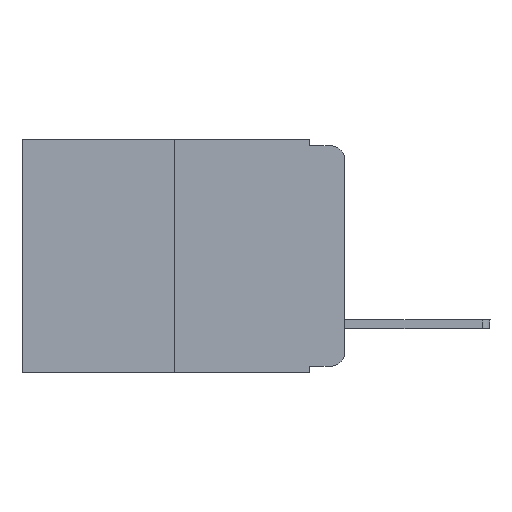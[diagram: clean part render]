
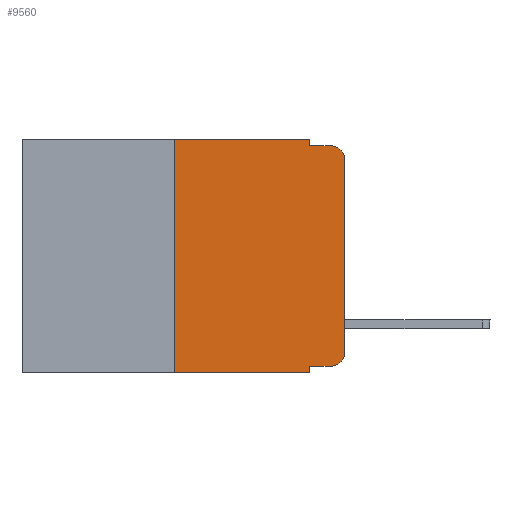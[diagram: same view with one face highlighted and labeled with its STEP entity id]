
A CAD part, left-side view. The second image highlights one B-rep face of the part: STEP entity #9560.
In plain terms, the highlighted planar face has unit normal (-1, 0, 0).
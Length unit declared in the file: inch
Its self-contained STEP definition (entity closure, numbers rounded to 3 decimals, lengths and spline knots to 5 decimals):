
#354 = LINE ( 'NONE', #13941, #14107 ) ;
#539 = CARTESIAN_POINT ( 'NONE',  ( 0., 0., -0.313 ) ) ;
#550 = ORIENTED_EDGE ( 'NONE', *, *, #10708, .F. ) ;
#658 = ORIENTED_EDGE ( 'NONE', *, *, #13967, .T. ) ;
#851 = VERTEX_POINT ( 'NONE', #7822 ) ;
#1199 = VECTOR ( 'NONE', #11061, 39.37008 ) ;
#1207 = CIRCLE ( 'NONE', #9537, 0.02 ) ;
#1257 = LINE ( 'NONE', #5520, #4127 ) ;
#1482 = LINE ( 'NONE', #12914, #13289 ) ;
#1785 = LINE ( 'NONE', #14321, #1199 ) ;
#2118 = DIRECTION ( 'NONE',  ( 0., -1., 0. ) ) ;
#2316 = DIRECTION ( 'NONE',  ( 0., 0., -1. ) ) ;
#2577 = DIRECTION ( 'NONE',  ( 0., -1., 0. ) ) ;
#2596 = DIRECTION ( 'NONE',  ( 0., 0., 1. ) ) ;
#2647 = EDGE_LOOP ( 'NONE', ( #3524, #3089, #8694, #12644, #550, #14440, #658, #9590, #8175, #4235 ) ) ;
#2706 = AXIS2_PLACEMENT_3D ( 'NONE', #4017, #4155, #7640 ) ;
#3079 = VERTEX_POINT ( 'NONE', #6579 ) ;
#3089 = ORIENTED_EDGE ( 'NONE', *, *, #12311, .T. ) ;
#3452 = DIRECTION ( 'NONE',  ( 0., 0., -1. ) ) ;
#3524 = ORIENTED_EDGE ( 'NONE', *, *, #10540, .T. ) ;
#3724 = LINE ( 'NONE', #10770, #3833 ) ;
#3833 = VECTOR ( 'NONE', #2596, 39.37008 ) ;
#4017 = CARTESIAN_POINT ( 'NONE',  ( 0., 0.02, -0.03 ) ) ;
#4127 = VECTOR ( 'NONE', #2316, 39.37008 ) ;
#4155 = DIRECTION ( 'NONE',  ( -1., 0., 0. ) ) ;
#4235 = ORIENTED_EDGE ( 'NONE', *, *, #9045, .T. ) ;
#4720 = FACE_OUTER_BOUND ( 'NONE', #2647, .T. ) ;
#4818 = LINE ( 'NONE', #13850, #9409 ) ;
#5110 = CARTESIAN_POINT ( 'NONE',  ( 0., 0.02, -0.01 ) ) ;
#5168 = VERTEX_POINT ( 'NONE', #10746 ) ;
#5216 = VERTEX_POINT ( 'NONE', #5110 ) ;
#5265 = CARTESIAN_POINT ( 'NONE',  ( 0., 0.051, -0.333 ) ) ;
#5301 = EDGE_CURVE ( 'NONE', #14570, #5216, #8800, .T. ) ;
#5520 = CARTESIAN_POINT ( 'NONE',  ( 0., 0.051, 0. ) ) ;
#6579 = CARTESIAN_POINT ( 'NONE',  ( 0., 0.051, -0.343 ) ) ;
#7280 = DIRECTION ( 'NONE',  ( 0., 0., 1. ) ) ;
#7375 = VECTOR ( 'NONE', #2118, 39.37008 ) ;
#7640 = DIRECTION ( 'NONE',  ( 0., 0., -1. ) ) ;
#7822 = CARTESIAN_POINT ( 'NONE',  ( 0., 0.051, -0.333 ) ) ;
#7926 = CIRCLE ( 'NONE', #2706, 0.02 ) ;
#8175 = ORIENTED_EDGE ( 'NONE', *, *, #14081, .T. ) ;
#8217 = AXIS2_PLACEMENT_3D ( 'NONE', #9246, #10437, #3452 ) ;
#8309 = DIRECTION ( 'NONE',  ( 0., 0., -1. ) ) ;
#8597 = LINE ( 'NONE', #5265, #13198 ) ;
#8694 = ORIENTED_EDGE ( 'NONE', *, *, #5301, .F. ) ;
#8703 = DIRECTION ( 'NONE',  ( -1., 0., 0. ) ) ;
#8800 = LINE ( 'NONE', #12353, #7375 ) ;
#9045 = EDGE_CURVE ( 'NONE', #5168, #14428, #1207, .T. ) ;
#9246 = CARTESIAN_POINT ( 'NONE',  ( 0., 0.473, 0. ) ) ;
#9409 = VECTOR ( 'NONE', #2577, 39.37008 ) ;
#9537 = AXIS2_PLACEMENT_3D ( 'NONE', #13223, #8703, #13155 ) ;
#9560 = ADVANCED_FACE ( 'NONE', ( #4720 ), #10360, .F. ) ;
#9590 = ORIENTED_EDGE ( 'NONE', *, *, #11569, .F. ) ;
#9931 = VERTEX_POINT ( 'NONE', #14357 ) ;
#10360 = PLANE ( 'NONE',  #8217 ) ;
#10437 = DIRECTION ( 'NONE',  ( 1., 0., 0. ) ) ;
#10540 = EDGE_CURVE ( 'NONE', #14428, #9931, #1482, .T. ) ;
#10612 = EDGE_CURVE ( 'NONE', #12064, #14503, #3724, .T. ) ;
#10708 = EDGE_CURVE ( 'NONE', #14503, #14584, #1785, .T. ) ;
#10746 = CARTESIAN_POINT ( 'NONE',  ( 0., 0.02, -0.333 ) ) ;
#10770 = CARTESIAN_POINT ( 'NONE',  ( 0., 0.25, 0. ) ) ;
#11016 = CARTESIAN_POINT ( 'NONE',  ( 0., 0.051, 0. ) ) ;
#11061 = DIRECTION ( 'NONE',  ( 0., -1., 0. ) ) ;
#11132 = CARTESIAN_POINT ( 'NONE',  ( 0., 0.25, -0.343 ) ) ;
#11569 = EDGE_CURVE ( 'NONE', #851, #3079, #1257, .T. ) ;
#12064 = VERTEX_POINT ( 'NONE', #11132 ) ;
#12127 = CARTESIAN_POINT ( 'NONE',  ( 0., 0.25, 0. ) ) ;
#12311 = EDGE_CURVE ( 'NONE', #9931, #5216, #7926, .T. ) ;
#12353 = CARTESIAN_POINT ( 'NONE',  ( 0., 0.051, -0.01 ) ) ;
#12644 = ORIENTED_EDGE ( 'NONE', *, *, #13390, .F. ) ;
#12914 = CARTESIAN_POINT ( 'NONE',  ( 0., 0., 0. ) ) ;
#13155 = DIRECTION ( 'NONE',  ( 0., 0., -1. ) ) ;
#13198 = VECTOR ( 'NONE', #14298, 39.37008 ) ;
#13223 = CARTESIAN_POINT ( 'NONE',  ( 0., 0.02, -0.313 ) ) ;
#13289 = VECTOR ( 'NONE', #7280, 39.37008 ) ;
#13390 = EDGE_CURVE ( 'NONE', #14584, #14570, #354, .T. ) ;
#13850 = CARTESIAN_POINT ( 'NONE',  ( 0., 0.473, -0.343 ) ) ;
#13941 = CARTESIAN_POINT ( 'NONE',  ( 0., 0.051, 0. ) ) ;
#13967 = EDGE_CURVE ( 'NONE', #12064, #3079, #4818, .T. ) ;
#14081 = EDGE_CURVE ( 'NONE', #851, #5168, #8597, .T. ) ;
#14107 = VECTOR ( 'NONE', #8309, 39.37008 ) ;
#14298 = DIRECTION ( 'NONE',  ( 0., -1., 0. ) ) ;
#14321 = CARTESIAN_POINT ( 'NONE',  ( 0., 0.473, 0. ) ) ;
#14357 = CARTESIAN_POINT ( 'NONE',  ( 0., 0., -0.03 ) ) ;
#14428 = VERTEX_POINT ( 'NONE', #539 ) ;
#14440 = ORIENTED_EDGE ( 'NONE', *, *, #10612, .F. ) ;
#14495 = CARTESIAN_POINT ( 'NONE',  ( 0., 0.051, -0.01 ) ) ;
#14503 = VERTEX_POINT ( 'NONE', #12127 ) ;
#14570 = VERTEX_POINT ( 'NONE', #14495 ) ;
#14584 = VERTEX_POINT ( 'NONE', #11016 ) ;
